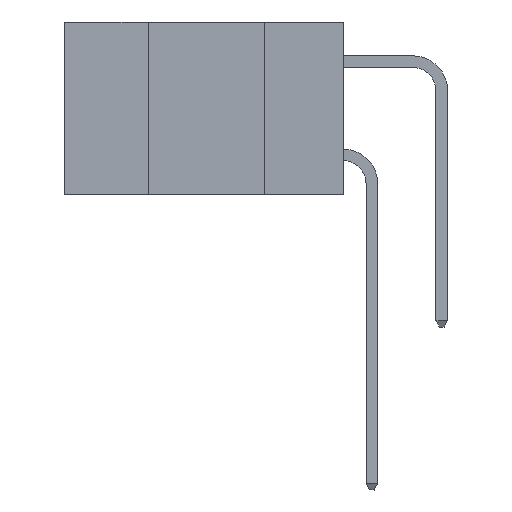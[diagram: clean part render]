
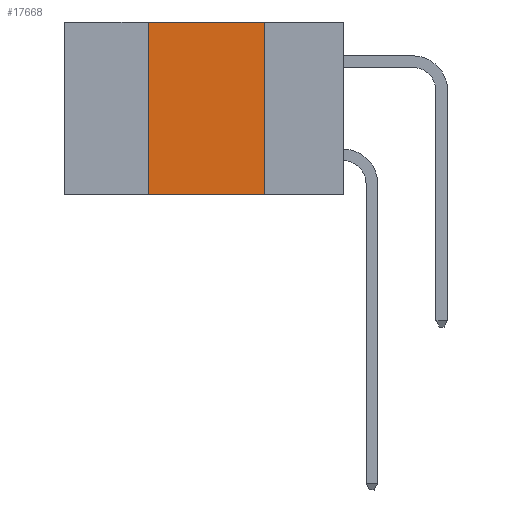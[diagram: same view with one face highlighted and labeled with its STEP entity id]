
A CAD part, left-side view. The second image highlights one B-rep face of the part: STEP entity #17668.
In plain terms, the highlighted planar face has unit normal (-1, 0, 0).
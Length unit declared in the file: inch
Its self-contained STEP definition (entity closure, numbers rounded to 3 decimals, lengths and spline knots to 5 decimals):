
#748 = EDGE_CURVE ( 'NONE', #5207, #14342, #17421, .T. ) ;
#1427 = LINE ( 'NONE', #8993, #21073 ) ;
#1629 = ORIENTED_EDGE ( 'NONE', *, *, #14950, .F. ) ;
#1729 = VECTOR ( 'NONE', #8341, 39.37008 ) ;
#4016 = DIRECTION ( 'NONE',  ( 0., 0., -1. ) ) ;
#4088 = ORIENTED_EDGE ( 'NONE', *, *, #9849, .F. ) ;
#5120 = CARTESIAN_POINT ( 'NONE',  ( 0., 0.17, 0. ) ) ;
#5207 = VERTEX_POINT ( 'NONE', #12124 ) ;
#5789 = DIRECTION ( 'NONE',  ( 0., -1., 0. ) ) ;
#5901 = ORIENTED_EDGE ( 'NONE', *, *, #748, .F. ) ;
#6959 = DIRECTION ( 'NONE',  ( 1., 0., 0. ) ) ;
#8341 = DIRECTION ( 'NONE',  ( 0., 0., 1. ) ) ;
#8993 = CARTESIAN_POINT ( 'NONE',  ( 0., 0.6, -0.37 ) ) ;
#9280 = EDGE_LOOP ( 'NONE', ( #4088, #1629, #5901, #19529 ) ) ;
#9570 = CARTESIAN_POINT ( 'NONE',  ( 0., 0.17, -0.37 ) ) ;
#9849 = EDGE_CURVE ( 'NONE', #15769, #22999, #20878, .T. ) ;
#12124 = CARTESIAN_POINT ( 'NONE',  ( 0., 0.42, -0.37 ) ) ;
#14340 = DIRECTION ( 'NONE',  ( 0., 0., -1. ) ) ;
#14342 = VERTEX_POINT ( 'NONE', #15598 ) ;
#14662 = LINE ( 'NONE', #21924, #20673 ) ;
#14950 = EDGE_CURVE ( 'NONE', #14342, #15769, #14662, .T. ) ;
#15392 = EDGE_CURVE ( 'NONE', #5207, #22999, #1427, .T. ) ;
#15598 = CARTESIAN_POINT ( 'NONE',  ( 0., 0.42, 0. ) ) ;
#15769 = VERTEX_POINT ( 'NONE', #5120 ) ;
#17421 = LINE ( 'NONE', #17555, #1729 ) ;
#17426 = VECTOR ( 'NONE', #4016, 39.37008 ) ;
#17555 = CARTESIAN_POINT ( 'NONE',  ( 0., 0.42, -0.37 ) ) ;
#17668 = ADVANCED_FACE ( 'NONE', ( #17794 ), #19756, .F. ) ;
#17794 = FACE_OUTER_BOUND ( 'NONE', #9280, .T. ) ;
#17922 = CARTESIAN_POINT ( 'NONE',  ( 0., 0.6, 0. ) ) ;
#17973 = DIRECTION ( 'NONE',  ( 0., -1., 0. ) ) ;
#19397 = CARTESIAN_POINT ( 'NONE',  ( 0., 0.17, -0.37 ) ) ;
#19529 = ORIENTED_EDGE ( 'NONE', *, *, #15392, .T. ) ;
#19756 = PLANE ( 'NONE',  #21545 ) ;
#20673 = VECTOR ( 'NONE', #5789, 39.37008 ) ;
#20878 = LINE ( 'NONE', #9570, #17426 ) ;
#21073 = VECTOR ( 'NONE', #17973, 39.37008 ) ;
#21545 = AXIS2_PLACEMENT_3D ( 'NONE', #17922, #6959, #14340 ) ;
#21924 = CARTESIAN_POINT ( 'NONE',  ( 0., 0.6, 0. ) ) ;
#22999 = VERTEX_POINT ( 'NONE', #19397 ) ;
